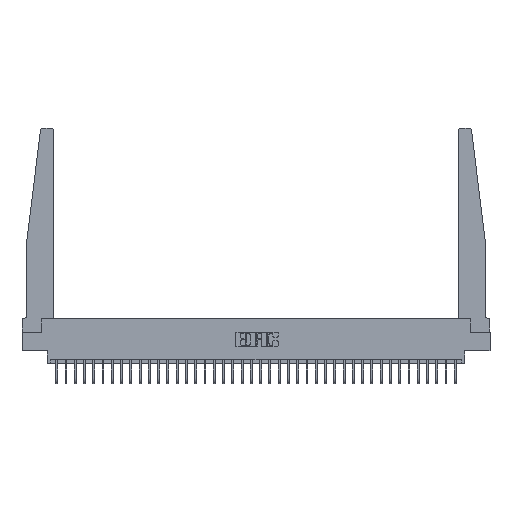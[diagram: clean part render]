
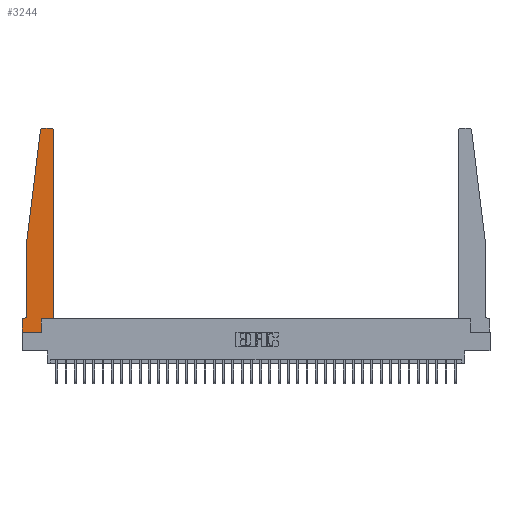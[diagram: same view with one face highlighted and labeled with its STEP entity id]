
A CAD part, top view. The second image highlights one B-rep face of the part: STEP entity #3244.
In plain terms, the highlighted planar face has unit normal (0, 0, 1).
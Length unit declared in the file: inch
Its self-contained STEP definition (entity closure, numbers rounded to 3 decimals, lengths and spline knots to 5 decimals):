
#591 = LINE ( 'NONE', #23425, #26116 ) ;
#623 = EDGE_CURVE ( 'NONE', #5532, #23427, #591, .T. ) ;
#892 = PLANE ( 'NONE',  #7977 ) ;
#1176 = DIRECTION ( 'NONE',  ( 1., 0., 0. ) ) ;
#1271 = DIRECTION ( 'NONE',  ( -1., 0., 0. ) ) ;
#1281 = EDGE_CURVE ( 'NONE', #28015, #2679, #22203, .T. ) ;
#2541 = ORIENTED_EDGE ( 'NONE', *, *, #20395, .T. ) ;
#2609 = ORIENTED_EDGE ( 'NONE', *, *, #6596, .T. ) ;
#2652 = CARTESIAN_POINT ( 'NONE',  ( 0.395, 2.75, 0.37 ) ) ;
#2679 = VERTEX_POINT ( 'NONE', #19212 ) ;
#2734 = ORIENTED_EDGE ( 'NONE', *, *, #30066, .T. ) ;
#3244 = ADVANCED_FACE ( 'NONE', ( #30563 ), #892, .T. ) ;
#3307 = VECTOR ( 'NONE', #28340, 39.37008 ) ;
#4146 = CARTESIAN_POINT ( 'NONE',  ( 0.27653, 2.72, 0.37 ) ) ;
#4702 = DIRECTION ( 'NONE',  ( 1., 0., 0. ) ) ;
#4715 = EDGE_CURVE ( 'NONE', #10889, #28015, #21582, .T. ) ;
#5532 = VERTEX_POINT ( 'NONE', #2652 ) ;
#5762 = ORIENTED_EDGE ( 'NONE', *, *, #26042, .T. ) ;
#6596 = EDGE_CURVE ( 'NONE', #2679, #25718, #15643, .T. ) ;
#6635 = DIRECTION ( 'NONE',  ( 1., 0., 0. ) ) ;
#6997 = VECTOR ( 'NONE', #8741, 39.37008 ) ;
#7216 = VERTEX_POINT ( 'NONE', #26670 ) ;
#7327 = DIRECTION ( 'NONE',  ( 0., 1., 0. ) ) ;
#7977 = AXIS2_PLACEMENT_3D ( 'NONE', #15670, #23159, #8383 ) ;
#8048 = ORIENTED_EDGE ( 'NONE', *, *, #17002, .T. ) ;
#8383 = DIRECTION ( 'NONE',  ( 1., 0., 0. ) ) ;
#8487 = VECTOR ( 'NONE', #28446, 39.37008 ) ;
#8741 = DIRECTION ( 'NONE',  ( 0., -1., 0. ) ) ;
#9229 = DIRECTION ( 'NONE',  ( 0., 0., -1. ) ) ;
#10806 = LINE ( 'NONE', #22271, #23181 ) ;
#10828 = ORIENTED_EDGE ( 'NONE', *, *, #4715, .T. ) ;
#10889 = VERTEX_POINT ( 'NONE', #24347 ) ;
#10920 = VERTEX_POINT ( 'NONE', #21951 ) ;
#11480 = DIRECTION ( 'NONE',  ( 0., 0., 1. ) ) ;
#11764 = LINE ( 'NONE', #30806, #30687 ) ;
#13277 = CARTESIAN_POINT ( 'NONE',  ( 0.425, 0.18, 0.37 ) ) ;
#13506 = DIRECTION ( 'NONE',  ( -1., 0., 0. ) ) ;
#13527 = CARTESIAN_POINT ( 'NONE',  ( 0.065, 1.25, 0.37 ) ) ;
#13647 = CARTESIAN_POINT ( 'NONE',  ( 0., 0., 0.37 ) ) ;
#14130 = CARTESIAN_POINT ( 'NONE',  ( 0., 0.1875, 0.37 ) ) ;
#15222 = LINE ( 'NONE', #27040, #27603 ) ;
#15643 = CIRCLE ( 'NONE', #27236, 0.05 ) ;
#15670 = CARTESIAN_POINT ( 'NONE',  ( 0., 0.1875, 0.37 ) ) ;
#15944 = CARTESIAN_POINT ( 'NONE',  ( 0., 0., 0.37 ) ) ;
#16063 = EDGE_LOOP ( 'NONE', ( #21300, #23653, #10828, #27729, #2609, #26890, #8048, #17516, #2734, #5762, #30377, #2541 ) ) ;
#16239 = VERTEX_POINT ( 'NONE', #13277 ) ;
#17002 = EDGE_CURVE ( 'NONE', #18359, #17843, #19303, .T. ) ;
#17516 = ORIENTED_EDGE ( 'NONE', *, *, #18850, .T. ) ;
#17843 = VERTEX_POINT ( 'NONE', #24379 ) ;
#18047 = CARTESIAN_POINT ( 'NONE',  ( 0.2605, 0., 0.37 ) ) ;
#18119 = CARTESIAN_POINT ( 'NONE',  ( 0.27653, 2.75, 0.37 ) ) ;
#18359 = VERTEX_POINT ( 'NONE', #14130 ) ;
#18548 = CARTESIAN_POINT ( 'NONE',  ( 0.065, 1.25, 0.37 ) ) ;
#18850 = EDGE_CURVE ( 'NONE', #17843, #28426, #26541, .T. ) ;
#18912 = VECTOR ( 'NONE', #4702, 39.37008 ) ;
#19212 = CARTESIAN_POINT ( 'NONE',  ( 0.065, 0.2375, 0.37 ) ) ;
#19303 = LINE ( 'NONE', #13647, #6997 ) ;
#20395 = EDGE_CURVE ( 'NONE', #7216, #5532, #28005, .T. ) ;
#20630 = EDGE_CURVE ( 'NONE', #16239, #7216, #15222, .T. ) ;
#21300 = ORIENTED_EDGE ( 'NONE', *, *, #623, .T. ) ;
#21360 = DIRECTION ( 'NONE',  ( 0., 0., 1. ) ) ;
#21582 = LINE ( 'NONE', #23603, #8487 ) ;
#21813 = AXIS2_PLACEMENT_3D ( 'NONE', #4146, #21360, #6635 ) ;
#21886 = LINE ( 'NONE', #21921, #18912 ) ;
#21921 = CARTESIAN_POINT ( 'NONE',  ( 0.425, 0.18, 0.37 ) ) ;
#21951 = CARTESIAN_POINT ( 'NONE',  ( 0.2605, 0.18, 0.37 ) ) ;
#22203 = LINE ( 'NONE', #13527, #3307 ) ;
#22271 = CARTESIAN_POINT ( 'NONE',  ( 0.2605, 0.18, 0.37 ) ) ;
#23145 = CARTESIAN_POINT ( 'NONE',  ( 0.015, 0.1875, 0.37 ) ) ;
#23159 = DIRECTION ( 'NONE',  ( 0., 0., 1. ) ) ;
#23181 = VECTOR ( 'NONE', #24774, 39.37008 ) ;
#23425 = CARTESIAN_POINT ( 'NONE',  ( 0.25, 2.75, 0.37 ) ) ;
#23427 = VERTEX_POINT ( 'NONE', #18119 ) ;
#23603 = CARTESIAN_POINT ( 'NONE',  ( 0.065, 1.25, 0.37 ) ) ;
#23653 = ORIENTED_EDGE ( 'NONE', *, *, #24780, .T. ) ;
#24006 = CARTESIAN_POINT ( 'NONE',  ( 0.015, 0.2375, 0.37 ) ) ;
#24048 = CIRCLE ( 'NONE', #21813, 0.03 ) ;
#24347 = CARTESIAN_POINT ( 'NONE',  ( 0.24675, 2.72367, 0.37 ) ) ;
#24379 = CARTESIAN_POINT ( 'NONE',  ( 0., 0., 0.37 ) ) ;
#24774 = DIRECTION ( 'NONE',  ( 0., 1., 0. ) ) ;
#24780 = EDGE_CURVE ( 'NONE', #23427, #10889, #24048, .T. ) ;
#25640 = AXIS2_PLACEMENT_3D ( 'NONE', #26291, #11480, #28750 ) ;
#25718 = VERTEX_POINT ( 'NONE', #23145 ) ;
#25764 = VECTOR ( 'NONE', #1176, 39.37008 ) ;
#26042 = EDGE_CURVE ( 'NONE', #10920, #16239, #21886, .T. ) ;
#26116 = VECTOR ( 'NONE', #1271, 39.37008 ) ;
#26291 = CARTESIAN_POINT ( 'NONE',  ( 0.395, 2.72, 0.37 ) ) ;
#26484 = DIRECTION ( 'NONE',  ( -1., 0., 0. ) ) ;
#26541 = LINE ( 'NONE', #15944, #25764 ) ;
#26670 = CARTESIAN_POINT ( 'NONE',  ( 0.425, 2.72, 0.37 ) ) ;
#26890 = ORIENTED_EDGE ( 'NONE', *, *, #29768, .T. ) ;
#27040 = CARTESIAN_POINT ( 'NONE',  ( 0.425, 0.18, 0.37 ) ) ;
#27236 = AXIS2_PLACEMENT_3D ( 'NONE', #24006, #9229, #26484 ) ;
#27603 = VECTOR ( 'NONE', #7327, 39.37008 ) ;
#27729 = ORIENTED_EDGE ( 'NONE', *, *, #1281, .T. ) ;
#28005 = CIRCLE ( 'NONE', #25640, 0.03 ) ;
#28015 = VERTEX_POINT ( 'NONE', #18548 ) ;
#28340 = DIRECTION ( 'NONE',  ( 0., -1., 0. ) ) ;
#28426 = VERTEX_POINT ( 'NONE', #18047 ) ;
#28446 = DIRECTION ( 'NONE',  ( -0.122, -0.992, 0. ) ) ;
#28750 = DIRECTION ( 'NONE',  ( 1., 0., 0. ) ) ;
#29768 = EDGE_CURVE ( 'NONE', #25718, #18359, #11764, .T. ) ;
#30066 = EDGE_CURVE ( 'NONE', #28426, #10920, #10806, .T. ) ;
#30377 = ORIENTED_EDGE ( 'NONE', *, *, #20630, .T. ) ;
#30563 = FACE_OUTER_BOUND ( 'NONE', #16063, .T. ) ;
#30687 = VECTOR ( 'NONE', #13506, 39.37008 ) ;
#30806 = CARTESIAN_POINT ( 'NONE',  ( 0.065, 0.1875, 0.37 ) ) ;
